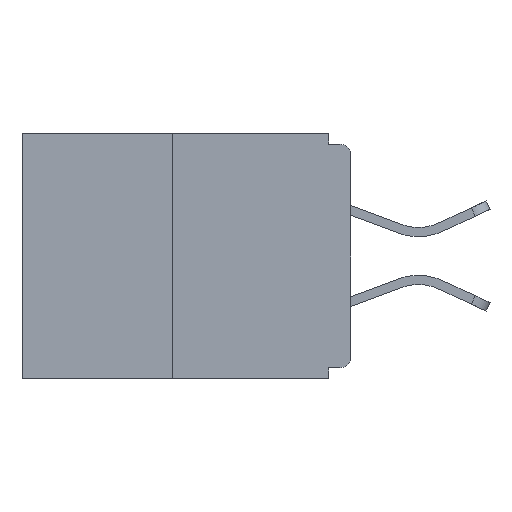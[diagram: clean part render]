
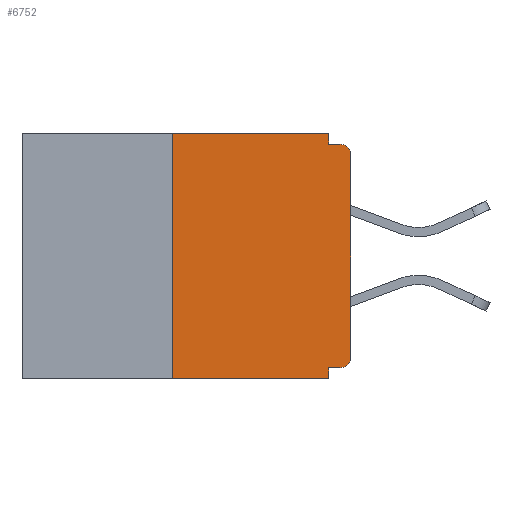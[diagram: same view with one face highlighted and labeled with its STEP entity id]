
A CAD part, left-side view. The second image highlights one B-rep face of the part: STEP entity #6752.
In plain terms, the highlighted planar face has unit normal (-1, 0, 0).
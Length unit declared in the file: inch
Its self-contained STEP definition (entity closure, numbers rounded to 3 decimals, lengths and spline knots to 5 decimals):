
#109 = DIRECTION ( 'NONE',  ( 0., 0., -1. ) ) ;
#265 = ORIENTED_EDGE ( 'NONE', *, *, #10864, .T. ) ;
#412 = DIRECTION ( 'NONE',  ( 0., 0., 1. ) ) ;
#825 = CARTESIAN_POINT ( 'NONE',  ( 0., 0.015, -0.015 ) ) ;
#1065 = VECTOR ( 'NONE', #9081, 39.37008 ) ;
#1211 = AXIS2_PLACEMENT_3D ( 'NONE', #7382, #8713, #5959 ) ;
#1244 = VERTEX_POINT ( 'NONE', #825 ) ;
#1249 = ORIENTED_EDGE ( 'NONE', *, *, #2364, .T. ) ;
#1405 = DIRECTION ( 'NONE',  ( 0., 0., -1. ) ) ;
#1987 = LINE ( 'NONE', #12403, #12058 ) ;
#2056 = VECTOR ( 'NONE', #109, 39.37008 ) ;
#2197 = VERTEX_POINT ( 'NONE', #7524 ) ;
#2364 = EDGE_CURVE ( 'NONE', #15298, #1244, #14638, .T. ) ;
#2636 = CARTESIAN_POINT ( 'NONE',  ( 0., 0.031, -0.343 ) ) ;
#3031 = DIRECTION ( 'NONE',  ( 0., -1., 0. ) ) ;
#3760 = DIRECTION ( 'NONE',  ( -1., 0., 0. ) ) ;
#3847 = LINE ( 'NONE', #15618, #12749 ) ;
#4319 = EDGE_CURVE ( 'NONE', #15106, #14259, #5621, .T. ) ;
#4462 = CARTESIAN_POINT ( 'NONE',  ( 0., 0.25, 0. ) ) ;
#4504 = CARTESIAN_POINT ( 'NONE',  ( 0., 0., -0.03 ) ) ;
#4861 = CARTESIAN_POINT ( 'NONE',  ( 0., 0.015, -0.03 ) ) ;
#4944 = CARTESIAN_POINT ( 'NONE',  ( 0., 0.031, 0. ) ) ;
#5066 = DIRECTION ( 'NONE',  ( -1., 0., 0. ) ) ;
#5144 = ORIENTED_EDGE ( 'NONE', *, *, #4319, .F. ) ;
#5237 = EDGE_CURVE ( 'NONE', #8700, #15106, #14289, .T. ) ;
#5292 = CARTESIAN_POINT ( 'NONE',  ( 0., 0.031, -0.328 ) ) ;
#5596 = CARTESIAN_POINT ( 'NONE',  ( 0., 0.031, -0.343 ) ) ;
#5602 = EDGE_CURVE ( 'NONE', #13065, #7052, #10722, .T. ) ;
#5621 = LINE ( 'NONE', #2636, #2056 ) ;
#5959 = DIRECTION ( 'NONE',  ( 0., 0., -1. ) ) ;
#6372 = EDGE_LOOP ( 'NONE', ( #6910, #11020, #265, #5144, #13186, #8204, #6629, #1249, #8239, #8041 ) ) ;
#6498 = CARTESIAN_POINT ( 'NONE',  ( 0., 0.015, -0.313 ) ) ;
#6620 = DIRECTION ( 'NONE',  ( 0., 1., 0. ) ) ;
#6629 = ORIENTED_EDGE ( 'NONE', *, *, #12417, .T. ) ;
#6752 = ADVANCED_FACE ( 'NONE', ( #13828 ), #7272, .F. ) ;
#6852 = AXIS2_PLACEMENT_3D ( 'NONE', #6498, #5066, #1405 ) ;
#6910 = ORIENTED_EDGE ( 'NONE', *, *, #13829, .F. ) ;
#6991 = VERTEX_POINT ( 'NONE', #4462 ) ;
#7052 = VERTEX_POINT ( 'NONE', #16046 ) ;
#7272 = PLANE ( 'NONE',  #1211 ) ;
#7382 = CARTESIAN_POINT ( 'NONE',  ( 0., 0.46, 0. ) ) ;
#7454 = DIRECTION ( 'NONE',  ( 0., 0., -1. ) ) ;
#7477 = DIRECTION ( 'NONE',  ( 0., 0., -1. ) ) ;
#7524 = CARTESIAN_POINT ( 'NONE',  ( 0., 0.25, -0.343 ) ) ;
#7742 = CARTESIAN_POINT ( 'NONE',  ( 0., 0., -0.015 ) ) ;
#7939 = CARTESIAN_POINT ( 'NONE',  ( 0., 0.25, 0. ) ) ;
#7955 = AXIS2_PLACEMENT_3D ( 'NONE', #4861, #3760, #7454 ) ;
#8022 = CARTESIAN_POINT ( 'NONE',  ( 0., 0.015, -0.328 ) ) ;
#8041 = ORIENTED_EDGE ( 'NONE', *, *, #5602, .F. ) ;
#8204 = ORIENTED_EDGE ( 'NONE', *, *, #10570, .T. ) ;
#8239 = ORIENTED_EDGE ( 'NONE', *, *, #12458, .F. ) ;
#8589 = DIRECTION ( 'NONE',  ( 0., -1., 0. ) ) ;
#8700 = VERTEX_POINT ( 'NONE', #8022 ) ;
#8713 = DIRECTION ( 'NONE',  ( 1., 0., 0. ) ) ;
#8951 = VERTEX_POINT ( 'NONE', #14613 ) ;
#8955 = CARTESIAN_POINT ( 'NONE',  ( 0., 0.031, 0. ) ) ;
#8960 = LINE ( 'NONE', #12897, #1065 ) ;
#9081 = DIRECTION ( 'NONE',  ( 0., 0., 1. ) ) ;
#9151 = LINE ( 'NONE', #7742, #15855 ) ;
#10570 = EDGE_CURVE ( 'NONE', #8700, #8951, #14915, .T. ) ;
#10722 = LINE ( 'NONE', #4944, #15836 ) ;
#10864 = EDGE_CURVE ( 'NONE', #2197, #14259, #3847, .T. ) ;
#11020 = ORIENTED_EDGE ( 'NONE', *, *, #15088, .F. ) ;
#11047 = LINE ( 'NONE', #7939, #13995 ) ;
#11341 = CARTESIAN_POINT ( 'NONE',  ( 0., 0., -0.328 ) ) ;
#11734 = DIRECTION ( 'NONE',  ( 0., -1., 0. ) ) ;
#12058 = VECTOR ( 'NONE', #8589, 39.37008 ) ;
#12403 = CARTESIAN_POINT ( 'NONE',  ( 0., 0.46, 0. ) ) ;
#12417 = EDGE_CURVE ( 'NONE', #8951, #15298, #8960, .T. ) ;
#12458 = EDGE_CURVE ( 'NONE', #7052, #1244, #9151, .T. ) ;
#12715 = VECTOR ( 'NONE', #6620, 39.37008 ) ;
#12749 = VECTOR ( 'NONE', #3031, 39.37008 ) ;
#12897 = CARTESIAN_POINT ( 'NONE',  ( 0., 0., 0. ) ) ;
#13065 = VERTEX_POINT ( 'NONE', #8955 ) ;
#13186 = ORIENTED_EDGE ( 'NONE', *, *, #5237, .F. ) ;
#13828 = FACE_OUTER_BOUND ( 'NONE', #6372, .T. ) ;
#13829 = EDGE_CURVE ( 'NONE', #6991, #13065, #1987, .T. ) ;
#13995 = VECTOR ( 'NONE', #412, 39.37008 ) ;
#14259 = VERTEX_POINT ( 'NONE', #5596 ) ;
#14289 = LINE ( 'NONE', #11341, #12715 ) ;
#14613 = CARTESIAN_POINT ( 'NONE',  ( 0., 0., -0.313 ) ) ;
#14638 = CIRCLE ( 'NONE', #7955, 0.015 ) ;
#14915 = CIRCLE ( 'NONE', #6852, 0.015 ) ;
#15088 = EDGE_CURVE ( 'NONE', #2197, #6991, #11047, .T. ) ;
#15106 = VERTEX_POINT ( 'NONE', #5292 ) ;
#15298 = VERTEX_POINT ( 'NONE', #4504 ) ;
#15618 = CARTESIAN_POINT ( 'NONE',  ( 0., 0.46, -0.343 ) ) ;
#15836 = VECTOR ( 'NONE', #7477, 39.37008 ) ;
#15855 = VECTOR ( 'NONE', #11734, 39.37008 ) ;
#16046 = CARTESIAN_POINT ( 'NONE',  ( 0., 0.031, -0.015 ) ) ;
